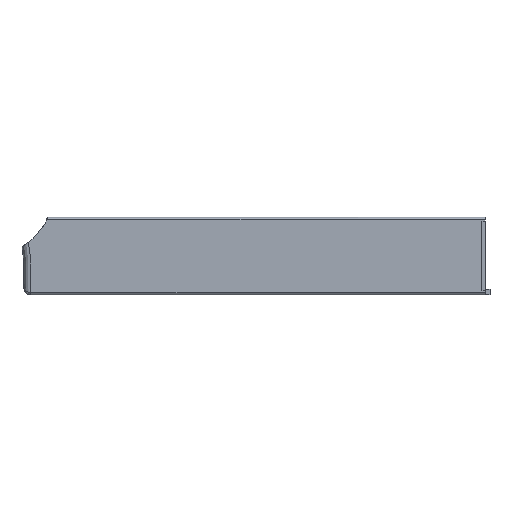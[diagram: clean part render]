
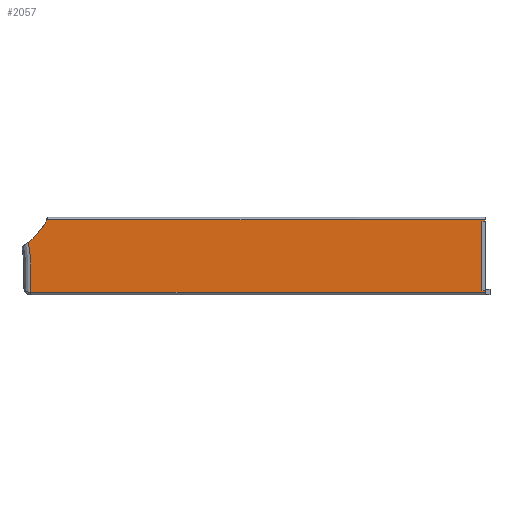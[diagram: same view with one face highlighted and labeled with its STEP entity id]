
A CAD part, left-side view. The second image highlights one B-rep face of the part: STEP entity #2057.
In plain terms, the highlighted planar face has unit normal (-1, 0, 0).
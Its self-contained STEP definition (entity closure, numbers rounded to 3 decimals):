
#13 = DIRECTION ( 'NONE',  ( 0., -0.281, 0.96 ) ) ;
#53 = CARTESIAN_POINT ( 'NONE',  ( -10.5, 196.971, -8.493 ) ) ;
#130 = ORIENTED_EDGE ( 'NONE', *, *, #5100, .T. ) ;
#168 = CARTESIAN_POINT ( 'NONE',  ( -10.5, 0., 15.05 ) ) ;
#190 = ORIENTED_EDGE ( 'NONE', *, *, #10977, .F. ) ;
#318 = EDGE_CURVE ( 'NONE', #10214, #8313, #9982, .T. ) ;
#369 = ORIENTED_EDGE ( 'NONE', *, *, #620, .F. ) ;
#620 = EDGE_CURVE ( 'NONE', #737, #5607, #1990, .T. ) ;
#698 = LINE ( 'NONE', #2399, #5178 ) ;
#737 = VERTEX_POINT ( 'NONE', #10021 ) ;
#842 = AXIS2_PLACEMENT_3D ( 'NONE', #1012, #1891, #8165 ) ;
#920 = CARTESIAN_POINT ( 'NONE',  ( -10.5, 195.137, -1.423 ) ) ;
#923 = VECTOR ( 'NONE', #2300, 1000. ) ;
#947 = LINE ( 'NONE', #4270, #3316 ) ;
#964 = CARTESIAN_POINT ( 'NONE',  ( -10.5, 196.992, -13.936 ) ) ;
#1012 = CARTESIAN_POINT ( 'NONE',  ( -10.5, 200., 0. ) ) ;
#1287 = ORIENTED_EDGE ( 'NONE', *, *, #7521, .F. ) ;
#1381 = LINE ( 'NONE', #7253, #6140 ) ;
#1382 = ORIENTED_EDGE ( 'NONE', *, *, #5579, .F. ) ;
#1648 = FACE_OUTER_BOUND ( 'NONE', #6629, .T. ) ;
#1722 = B_SPLINE_CURVE_WITH_KNOTS ( 'NONE', 3,
 ( #9692, #5379, #7190, #1802, #8071, #2712, #8966, #3620, #9872, #4516, #10790, #5423, #53, #6333, #964, #7226 ),
 .UNSPECIFIED., .F., .F.,
 ( 4, 2, 2, 2, 2, 2, 2, 4 ),
 ( 0., 0.003, 0.005, 0.008, 0.01, 0.011, 0.016, 0.022 ),
 .UNSPECIFIED. ) ;
#1802 = CARTESIAN_POINT ( 'NONE',  ( -10.5, 197.568, 2.355 ) ) ;
#1891 = DIRECTION ( 'NONE',  ( -1., 0., 0. ) ) ;
#1990 = LINE ( 'NONE', #4108, #3822 ) ;
#2015 = CARTESIAN_POINT ( 'NONE',  ( -10.5, 196., 7.503 ) ) ;
#2057 = ADVANCED_FACE ( 'NONE', ( #1648 ), #9925, .T. ) ;
#2285 = ORIENTED_EDGE ( 'NONE', *, *, #318, .F. ) ;
#2300 = DIRECTION ( 'NONE',  ( 0., -1., 0. ) ) ;
#2377 = ORIENTED_EDGE ( 'NONE', *, *, #10638, .F. ) ;
#2399 = CARTESIAN_POINT ( 'NONE',  ( -10.5, 200., -15.75 ) ) ;
#2408 = CARTESIAN_POINT ( 'NONE',  ( -10.5, 190.111, 15.75 ) ) ;
#2700 = DIRECTION ( 'NONE',  ( 0., 1., 0. ) ) ;
#2712 = CARTESIAN_POINT ( 'NONE',  ( -10.5, 197.187, -0.341 ) ) ;
#3077 = EDGE_CURVE ( 'NONE', #10214, #6039, #1381, .T. ) ;
#3105 = VECTOR ( 'NONE', #13, 1000. ) ;
#3118 = VECTOR ( 'NONE', #4106, 1000. ) ;
#3184 = VECTOR ( 'NONE', #5112, 1000. ) ;
#3213 = DIRECTION ( 'NONE',  ( 0., 0., -1. ) ) ;
#3302 = DIRECTION ( 'NONE',  ( 0., -1., 0. ) ) ;
#3316 = VECTOR ( 'NONE', #5175, 1000. ) ;
#3620 = CARTESIAN_POINT ( 'NONE',  ( -10.5, 196.988, -2.597 ) ) ;
#3822 = VECTOR ( 'NONE', #3213, 1000. ) ;
#4079 = LINE ( 'NONE', #5211, #6182 ) ;
#4106 = DIRECTION ( 'NONE',  ( 0., 0., -1. ) ) ;
#4108 = CARTESIAN_POINT ( 'NONE',  ( -10.5, 1.5, 0. ) ) ;
#4270 = CARTESIAN_POINT ( 'NONE',  ( -10.5, 201.302, 1.074 ) ) ;
#4313 = VERTEX_POINT ( 'NONE', #7775 ) ;
#4516 = CARTESIAN_POINT ( 'NONE',  ( -10.5, 196.964, -3.957 ) ) ;
#4586 = EDGE_CURVE ( 'NONE', #6292, #9657, #947, .T. ) ;
#4616 = CARTESIAN_POINT ( 'NONE',  ( -10.5, 190.613, 14.036 ) ) ;
#5072 = VERTEX_POINT ( 'NONE', #7900 ) ;
#5100 = EDGE_CURVE ( 'NONE', #7344, #4313, #1722, .T. ) ;
#5112 = DIRECTION ( 'NONE',  ( 0., -1., 0. ) ) ;
#5175 = DIRECTION ( 'NONE',  ( 0., -0.636, 0.771 ) ) ;
#5178 = VECTOR ( 'NONE', #3302, 1000. ) ;
#5211 = CARTESIAN_POINT ( 'NONE',  ( -10.5, 202.161, 2.879 ) ) ;
#5379 = CARTESIAN_POINT ( 'NONE',  ( -10.5, 197.945, 5.052 ) ) ;
#5423 = CARTESIAN_POINT ( 'NONE',  ( -10.5, 196.96, -6.678 ) ) ;
#5488 = LINE ( 'NONE', #5947, #5773 ) ;
#5579 = EDGE_CURVE ( 'NONE', #5607, #5072, #8229, .T. ) ;
#5607 = VERTEX_POINT ( 'NONE', #6926 ) ;
#5773 = VECTOR ( 'NONE', #6849, 1000. ) ;
#5947 = CARTESIAN_POINT ( 'NONE',  ( -10.5, 200., -15.75 ) ) ;
#5973 = VERTEX_POINT ( 'NONE', #9426 ) ;
#6039 = VERTEX_POINT ( 'NONE', #2408 ) ;
#6110 = VERTEX_POINT ( 'NONE', #11495 ) ;
#6140 = VECTOR ( 'NONE', #2700, 1000. ) ;
#6182 = VECTOR ( 'NONE', #10579, 1000. ) ;
#6221 = CARTESIAN_POINT ( 'NONE',  ( -10.5, 0., 15.75 ) ) ;
#6292 = VERTEX_POINT ( 'NONE', #2015 ) ;
#6333 = CARTESIAN_POINT ( 'NONE',  ( -10.5, 196.985, -12.121 ) ) ;
#6629 = EDGE_LOOP ( 'NONE', ( #190, #130, #8082, #7640, #1287, #1382, #369, #7264, #2285, #6688, #2377, #7957 ) ) ;
#6688 = ORIENTED_EDGE ( 'NONE', *, *, #3077, .T. ) ;
#6849 = DIRECTION ( 'NONE',  ( 0., -1., 0. ) ) ;
#6926 = CARTESIAN_POINT ( 'NONE',  ( -10.5, 1.5, -15.05 ) ) ;
#7114 = EDGE_CURVE ( 'NONE', #737, #8313, #10176, .T. ) ;
#7190 = CARTESIAN_POINT ( 'NONE',  ( -10.5, 197.821, 4.152 ) ) ;
#7226 = CARTESIAN_POINT ( 'NONE',  ( -10.5, 196.997, -15.75 ) ) ;
#7253 = CARTESIAN_POINT ( 'NONE',  ( -10.5, 189.818, 15.75 ) ) ;
#7264 = ORIENTED_EDGE ( 'NONE', *, *, #7114, .T. ) ;
#7344 = VERTEX_POINT ( 'NONE', #8211 ) ;
#7521 = EDGE_CURVE ( 'NONE', #5072, #5973, #8483, .T. ) ;
#7640 = ORIENTED_EDGE ( 'NONE', *, *, #11404, .T. ) ;
#7775 = CARTESIAN_POINT ( 'NONE',  ( -10.5, 196.997, -15.75 ) ) ;
#7900 = CARTESIAN_POINT ( 'NONE',  ( -10.5, 0., -15.05 ) ) ;
#7957 = ORIENTED_EDGE ( 'NONE', *, *, #4586, .F. ) ;
#8071 = CARTESIAN_POINT ( 'NONE',  ( -10.5, 197.437, 1.457 ) ) ;
#8082 = ORIENTED_EDGE ( 'NONE', *, *, #11491, .T. ) ;
#8165 = DIRECTION ( 'NONE',  ( 0., 0., 1. ) ) ;
#8205 = VECTOR ( 'NONE', #9374, 1000. ) ;
#8211 = CARTESIAN_POINT ( 'NONE',  ( -10.5, 198.068, 5.951 ) ) ;
#8229 = LINE ( 'NONE', #8680, #3184 ) ;
#8313 = VERTEX_POINT ( 'NONE', #168 ) ;
#8475 = CARTESIAN_POINT ( 'NONE',  ( -10.5, 0., 0. ) ) ;
#8483 = LINE ( 'NONE', #8475, #8205 ) ;
#8680 = CARTESIAN_POINT ( 'NONE',  ( -10.5, 1.5, -15.05 ) ) ;
#8966 = CARTESIAN_POINT ( 'NONE',  ( -10.5, 197.068, -1.241 ) ) ;
#9374 = DIRECTION ( 'NONE',  ( 0., 0., -1. ) ) ;
#9426 = CARTESIAN_POINT ( 'NONE',  ( -10.5, 0., -15.75 ) ) ;
#9657 = VERTEX_POINT ( 'NONE', #4616 ) ;
#9692 = CARTESIAN_POINT ( 'NONE',  ( -10.5, 198.068, 5.951 ) ) ;
#9872 = CARTESIAN_POINT ( 'NONE',  ( -10.5, 196.977, -3.05 ) ) ;
#9925 = PLANE ( 'NONE',  #842 ) ;
#9982 = LINE ( 'NONE', #11274, #3118 ) ;
#10021 = CARTESIAN_POINT ( 'NONE',  ( -10.5, 1.5, 15.05 ) ) ;
#10176 = LINE ( 'NONE', #10298, #923 ) ;
#10214 = VERTEX_POINT ( 'NONE', #6221 ) ;
#10254 = LINE ( 'NONE', #920, #3105 ) ;
#10298 = CARTESIAN_POINT ( 'NONE',  ( -10.5, 1.5, 15.05 ) ) ;
#10579 = DIRECTION ( 'NONE',  ( 0., -0.8, 0.6 ) ) ;
#10638 = EDGE_CURVE ( 'NONE', #9657, #6039, #10254, .T. ) ;
#10790 = CARTESIAN_POINT ( 'NONE',  ( -10.5, 196.963, -4.41 ) ) ;
#10977 = EDGE_CURVE ( 'NONE', #7344, #6292, #4079, .T. ) ;
#11274 = CARTESIAN_POINT ( 'NONE',  ( -10.5, 0., 0. ) ) ;
#11404 = EDGE_CURVE ( 'NONE', #6110, #5973, #5488, .T. ) ;
#11491 = EDGE_CURVE ( 'NONE', #4313, #6110, #698, .T. ) ;
#11495 = CARTESIAN_POINT ( 'NONE',  ( -10.5, 196.991, -15.75 ) ) ;
